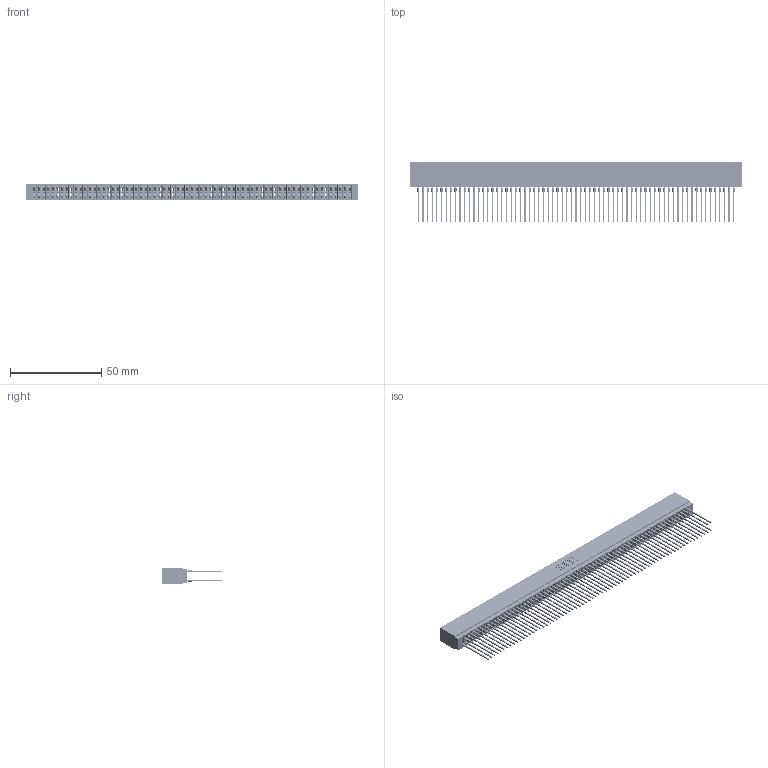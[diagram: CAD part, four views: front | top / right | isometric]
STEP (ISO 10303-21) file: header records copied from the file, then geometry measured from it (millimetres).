
FILE_DESCRIPTION (( 'STEP AP203' ), '1' );
FILE_NAME ('725-138-541-201.STEP', '2026-02-25T21:37:58', ( '' ), ( '' ), 'SwSTEP 2.0', 'SolidWorks 2023', '' );
FILE_SCHEMA (( 'CONFIG_CONTROL_DESIGN' ));
Length unit declared in the file: millimetre
Products named in the file (3): 745-292-001_541; 725-138-541-201; 725 Part_Insulator Option - 01
Assembly tree (139 placements, depth 2):
  725-138-541-201
    725 Part_Insulator Option - 01
    745-292-001_541  x138
Bounding box: 181.86 x 33.03 x 8.89 mm (x, y, z)
Volume: 14962.2 mm3; surface area: 34907.5 mm2
Topology: 139 solids, 139 shells, 12446 faces, 33443 edges, 21006 vertices
Faces by surface type: plane 6403, bspline 2760, cylinder 2455, torus 828
Entity records: 112441 total; most frequent: CARTESIAN_POINT 19995, ORIENTED_EDGE 19484, DIRECTION 17000, EDGE_CURVE 9742, LINE 9146, VECTOR 9146, VERTEX_POINT 6210, AXIS2_PLACEMENT_3D 3927
